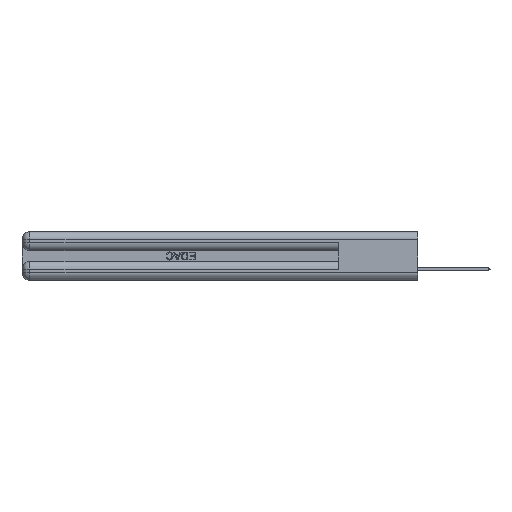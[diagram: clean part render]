
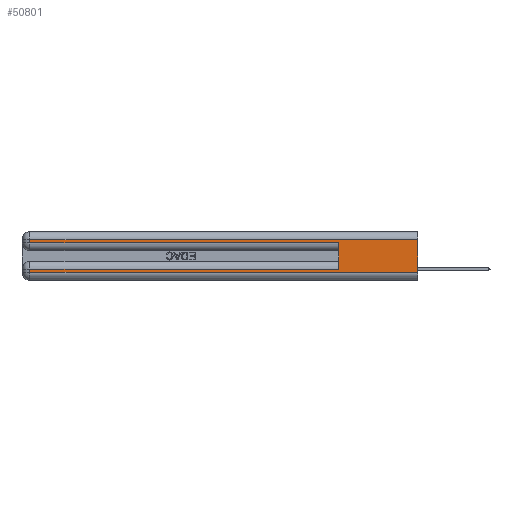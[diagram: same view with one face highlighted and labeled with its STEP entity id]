
A CAD part, left-side view. The second image highlights one B-rep face of the part: STEP entity #50801.
In plain terms, the highlighted planar face has unit normal (-1, 0, 0).
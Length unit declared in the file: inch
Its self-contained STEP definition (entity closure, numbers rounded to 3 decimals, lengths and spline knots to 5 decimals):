
#419 = EDGE_LOOP ( 'NONE', ( #37367, #14148, #47405, #428, #20227, #34429, #42839, #49569 ) ) ;
#428 = ORIENTED_EDGE ( 'NONE', *, *, #28237, .T. ) ;
#429 = VERTEX_POINT ( 'NONE', #4948 ) ;
#1501 = VERTEX_POINT ( 'NONE', #5826 ) ;
#2536 = DIRECTION ( 'NONE',  ( 0., 0., -1. ) ) ;
#3495 = DIRECTION ( 'NONE',  ( 0., 0., -1. ) ) ;
#4948 = CARTESIAN_POINT ( 'NONE',  ( 0., 0., 0.06 ) ) ;
#5518 = CARTESIAN_POINT ( 'NONE',  ( 0., 2.94, 0.06 ) ) ;
#5826 = CARTESIAN_POINT ( 'NONE',  ( 0., 2.94, 0.285 ) ) ;
#6029 = CARTESIAN_POINT ( 'NONE',  ( 0., 0., 0.31 ) ) ;
#7187 = VECTOR ( 'NONE', #41473, 39.37008 ) ;
#7989 = EDGE_CURVE ( 'NONE', #37949, #429, #33822, .T. ) ;
#8684 = VERTEX_POINT ( 'NONE', #54220 ) ;
#10747 = EDGE_CURVE ( 'NONE', #37692, #429, #34484, .T. ) ;
#11344 = CARTESIAN_POINT ( 'NONE',  ( 0., 0.6, 0.085 ) ) ;
#11601 = CARTESIAN_POINT ( 'NONE',  ( 0., 0., 0.285 ) ) ;
#12747 = EDGE_CURVE ( 'NONE', #8684, #1501, #15765, .T. ) ;
#13215 = VECTOR ( 'NONE', #49486, 39.37008 ) ;
#13384 = CARTESIAN_POINT ( 'NONE',  ( 0., 2.94, 0.085 ) ) ;
#14148 = ORIENTED_EDGE ( 'NONE', *, *, #16014, .T. ) ;
#15765 = LINE ( 'NONE', #41204, #25001 ) ;
#16014 = EDGE_CURVE ( 'NONE', #37692, #8684, #52305, .T. ) ;
#18125 = LINE ( 'NONE', #52028, #38606 ) ;
#20227 = ORIENTED_EDGE ( 'NONE', *, *, #38237, .F. ) ;
#25001 = VECTOR ( 'NONE', #2536, 39.37008 ) ;
#26983 = VECTOR ( 'NONE', #45703, 39.37008 ) ;
#27717 = DIRECTION ( 'NONE',  ( 0., 1., 0. ) ) ;
#27812 = DIRECTION ( 'NONE',  ( 0., 0., -1. ) ) ;
#28237 = EDGE_CURVE ( 'NONE', #1501, #47577, #34892, .T. ) ;
#29749 = CARTESIAN_POINT ( 'NONE',  ( 0., 0., 0.31 ) ) ;
#30083 = VECTOR ( 'NONE', #53289, 39.37008 ) ;
#32051 = CARTESIAN_POINT ( 'NONE',  ( 0., 2.94, 0.37 ) ) ;
#33320 = VECTOR ( 'NONE', #27717, 39.37008 ) ;
#33468 = FACE_OUTER_BOUND ( 'NONE', #419, .T. ) ;
#33542 = VERTEX_POINT ( 'NONE', #11344 ) ;
#33822 = LINE ( 'NONE', #49094, #13215 ) ;
#34429 = ORIENTED_EDGE ( 'NONE', *, *, #46237, .T. ) ;
#34484 = LINE ( 'NONE', #40881, #44304 ) ;
#34892 = LINE ( 'NONE', #11601, #7187 ) ;
#37135 = DIRECTION ( 'NONE',  ( 1., 0., 0. ) ) ;
#37367 = ORIENTED_EDGE ( 'NONE', *, *, #10747, .F. ) ;
#37692 = VERTEX_POINT ( 'NONE', #29749 ) ;
#37949 = VERTEX_POINT ( 'NONE', #5518 ) ;
#38237 = EDGE_CURVE ( 'NONE', #33542, #47577, #52719, .T. ) ;
#38606 = VECTOR ( 'NONE', #42191, 39.37008 ) ;
#40881 = CARTESIAN_POINT ( 'NONE',  ( 0., 0., 0.37 ) ) ;
#41149 = PLANE ( 'NONE',  #52094 ) ;
#41204 = CARTESIAN_POINT ( 'NONE',  ( 0., 2.94, 0.37 ) ) ;
#41473 = DIRECTION ( 'NONE',  ( 0., -1., 0. ) ) ;
#41809 = VERTEX_POINT ( 'NONE', #13384 ) ;
#42191 = DIRECTION ( 'NONE',  ( 0., 1., 0. ) ) ;
#42839 = ORIENTED_EDGE ( 'NONE', *, *, #46115, .T. ) ;
#44304 = VECTOR ( 'NONE', #27812, 39.37008 ) ;
#45703 = DIRECTION ( 'NONE',  ( 0., 0., 1. ) ) ;
#46115 = EDGE_CURVE ( 'NONE', #41809, #37949, #49226, .T. ) ;
#46237 = EDGE_CURVE ( 'NONE', #33542, #41809, #18125, .T. ) ;
#47405 = ORIENTED_EDGE ( 'NONE', *, *, #12747, .T. ) ;
#47577 = VERTEX_POINT ( 'NONE', #52684 ) ;
#49094 = CARTESIAN_POINT ( 'NONE',  ( 0., 0., 0.06 ) ) ;
#49226 = LINE ( 'NONE', #32051, #30083 ) ;
#49486 = DIRECTION ( 'NONE',  ( 0., -1., 0. ) ) ;
#49569 = ORIENTED_EDGE ( 'NONE', *, *, #7989, .T. ) ;
#50801 = ADVANCED_FACE ( 'NONE', ( #33468 ), #41149, .F. ) ;
#52028 = CARTESIAN_POINT ( 'NONE',  ( 0., 0., 0.085 ) ) ;
#52094 = AXIS2_PLACEMENT_3D ( 'NONE', #54105, #37135, #3495 ) ;
#52305 = LINE ( 'NONE', #6029, #33320 ) ;
#52684 = CARTESIAN_POINT ( 'NONE',  ( 0., 0.6, 0.285 ) ) ;
#52719 = LINE ( 'NONE', #54002, #26983 ) ;
#53289 = DIRECTION ( 'NONE',  ( 0., 0., -1. ) ) ;
#54002 = CARTESIAN_POINT ( 'NONE',  ( 0., 0.6, 0.145 ) ) ;
#54105 = CARTESIAN_POINT ( 'NONE',  ( 0., 0., 0.37 ) ) ;
#54220 = CARTESIAN_POINT ( 'NONE',  ( 0., 2.94, 0.31 ) ) ;
